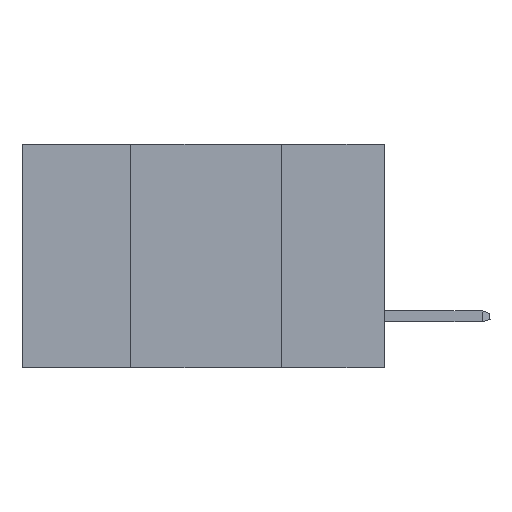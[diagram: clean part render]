
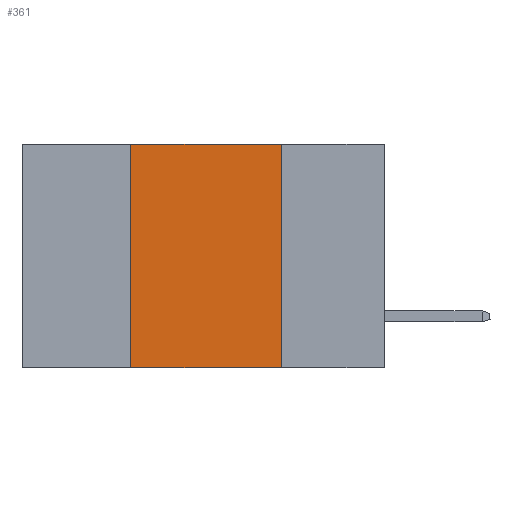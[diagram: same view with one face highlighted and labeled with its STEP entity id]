
A CAD part, left-side view. The second image highlights one B-rep face of the part: STEP entity #361.
In plain terms, the highlighted planar face has unit normal (-1, 0, 0).
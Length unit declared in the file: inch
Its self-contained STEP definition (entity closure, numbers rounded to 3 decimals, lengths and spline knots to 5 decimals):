
#154 = FACE_OUTER_BOUND ( 'NONE', #5749, .T. ) ;
#299 = CARTESIAN_POINT ( 'NONE',  ( 0., 0.42, 0. ) ) ;
#361 = ADVANCED_FACE ( 'NONE', ( #154 ), #12103, .F. ) ;
#662 = LINE ( 'NONE', #2951, #3049 ) ;
#1643 = ORIENTED_EDGE ( 'NONE', *, *, #3910, .F. ) ;
#1683 = VECTOR ( 'NONE', #7662, 39.37008 ) ;
#1874 = EDGE_CURVE ( 'NONE', #4283, #2285, #13697, .T. ) ;
#1973 = CARTESIAN_POINT ( 'NONE',  ( 0., 0.17, -0.37 ) ) ;
#2285 = VERTEX_POINT ( 'NONE', #1973 ) ;
#2951 = CARTESIAN_POINT ( 'NONE',  ( 0., 0.17, 0. ) ) ;
#3049 = VECTOR ( 'NONE', #8572, 39.37008 ) ;
#3181 = DIRECTION ( 'NONE',  ( 0., 0., 1. ) ) ;
#3236 = CARTESIAN_POINT ( 'NONE',  ( 0., 0.42, 0. ) ) ;
#3335 = CARTESIAN_POINT ( 'NONE',  ( 0., 0.6, 0. ) ) ;
#3450 = CARTESIAN_POINT ( 'NONE',  ( 0., 0.6, 0. ) ) ;
#3910 = EDGE_CURVE ( 'NONE', #4283, #6298, #7558, .T. ) ;
#4283 = VERTEX_POINT ( 'NONE', #5543 ) ;
#4532 = CARTESIAN_POINT ( 'NONE',  ( 0., 0.17, 0. ) ) ;
#5476 = EDGE_CURVE ( 'NONE', #7485, #2285, #662, .T. ) ;
#5486 = ORIENTED_EDGE ( 'NONE', *, *, #1874, .T. ) ;
#5525 = EDGE_CURVE ( 'NONE', #6298, #7485, #6826, .T. ) ;
#5543 = CARTESIAN_POINT ( 'NONE',  ( 0., 0.42, -0.37 ) ) ;
#5749 = EDGE_LOOP ( 'NONE', ( #10843, #10457, #1643, #5486 ) ) ;
#5978 = AXIS2_PLACEMENT_3D ( 'NONE', #3450, #13211, #6600 ) ;
#6298 = VERTEX_POINT ( 'NONE', #299 ) ;
#6600 = DIRECTION ( 'NONE',  ( 0., 0., -1. ) ) ;
#6826 = LINE ( 'NONE', #3335, #1683 ) ;
#7485 = VERTEX_POINT ( 'NONE', #4532 ) ;
#7558 = LINE ( 'NONE', #3236, #8770 ) ;
#7662 = DIRECTION ( 'NONE',  ( 0., -1., 0. ) ) ;
#7850 = VECTOR ( 'NONE', #10138, 39.37008 ) ;
#8572 = DIRECTION ( 'NONE',  ( 0., 0., -1. ) ) ;
#8770 = VECTOR ( 'NONE', #3181, 39.37008 ) ;
#10138 = DIRECTION ( 'NONE',  ( 0., -1., 0. ) ) ;
#10457 = ORIENTED_EDGE ( 'NONE', *, *, #5525, .F. ) ;
#10843 = ORIENTED_EDGE ( 'NONE', *, *, #5476, .F. ) ;
#12103 = PLANE ( 'NONE',  #5978 ) ;
#12148 = CARTESIAN_POINT ( 'NONE',  ( 0., 0.6, -0.37 ) ) ;
#13211 = DIRECTION ( 'NONE',  ( 1., 0., 0. ) ) ;
#13697 = LINE ( 'NONE', #12148, #7850 ) ;
